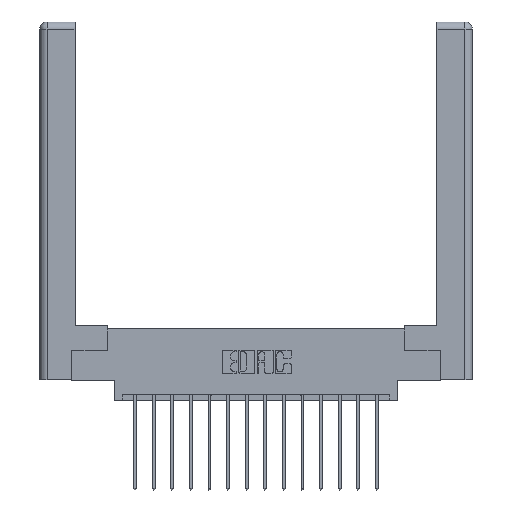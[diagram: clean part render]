
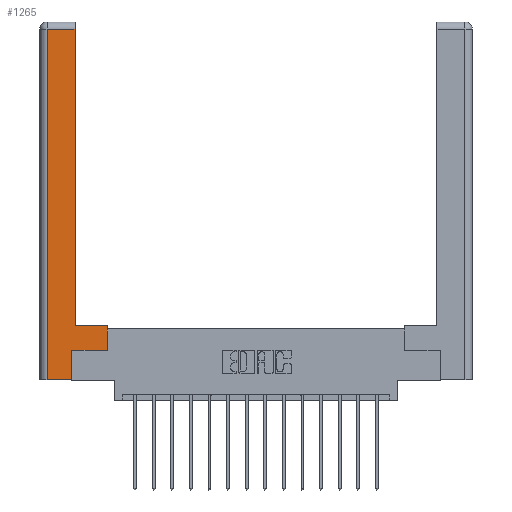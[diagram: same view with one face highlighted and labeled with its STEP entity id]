
A CAD part, top view. The second image highlights one B-rep face of the part: STEP entity #1265.
In plain terms, the highlighted planar face has unit normal (0, 0, 1).
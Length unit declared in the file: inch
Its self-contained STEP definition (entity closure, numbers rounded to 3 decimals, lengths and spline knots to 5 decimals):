
#77 = CARTESIAN_POINT ( 'NONE',  ( 0.0615, 0., 0. ) ) ;
#133 = FACE_OUTER_BOUND ( 'NONE', #11661, .T. ) ;
#338 = VECTOR ( 'NONE', #8718, 39.37008 ) ;
#822 = EDGE_CURVE ( 'NONE', #15724, #2170, #10951, .T. ) ;
#1139 = EDGE_CURVE ( 'NONE', #3528, #12792, #16197, .T. ) ;
#1265 = ADVANCED_FACE ( 'NONE', ( #133 ), #13441, .F. ) ;
#1387 = AXIS2_PLACEMENT_3D ( 'NONE', #4194, #10757, #2815 ) ;
#1439 = ORIENTED_EDGE ( 'NONE', *, *, #4792, .T. ) ;
#1557 = DIRECTION ( 'NONE',  ( 0., 1., 0. ) ) ;
#1636 = CARTESIAN_POINT ( 'NONE',  ( 0.565, 0.245, 0. ) ) ;
#1803 = VECTOR ( 'NONE', #3626, 39.37008 ) ;
#1825 = CARTESIAN_POINT ( 'NONE',  ( 0.265, 0.245, 0. ) ) ;
#2148 = VERTEX_POINT ( 'NONE', #11118 ) ;
#2170 = VERTEX_POINT ( 'NONE', #11792 ) ;
#2693 = CARTESIAN_POINT ( 'NONE',  ( 0.0615, 2.94, 0. ) ) ;
#2815 = DIRECTION ( 'NONE',  ( -1., 0., 0. ) ) ;
#2923 = DIRECTION ( 'NONE',  ( 1., 0., 0. ) ) ;
#3528 = VERTEX_POINT ( 'NONE', #2693 ) ;
#3626 = DIRECTION ( 'NONE',  ( 1., 0., 0. ) ) ;
#3769 = DIRECTION ( 'NONE',  ( 0., -1., 0. ) ) ;
#4194 = CARTESIAN_POINT ( 'NONE',  ( 0., 0., 0. ) ) ;
#4705 = ORIENTED_EDGE ( 'NONE', *, *, #16252, .T. ) ;
#4792 = EDGE_CURVE ( 'NONE', #7617, #15724, #8125, .T. ) ;
#5646 = DIRECTION ( 'NONE',  ( 0., 1., 0. ) ) ;
#6148 = LINE ( 'NONE', #6435, #1803 ) ;
#6435 = CARTESIAN_POINT ( 'NONE',  ( 0.265, 0., 0. ) ) ;
#6750 = VECTOR ( 'NONE', #3769, 39.37008 ) ;
#6788 = ORIENTED_EDGE ( 'NONE', *, *, #10988, .T. ) ;
#7175 = VECTOR ( 'NONE', #16006, 39.37008 ) ;
#7399 = DIRECTION ( 'NONE',  ( 0., 1., 0. ) ) ;
#7617 = VERTEX_POINT ( 'NONE', #1825 ) ;
#8019 = EDGE_CURVE ( 'NONE', #2170, #9097, #10737, .T. ) ;
#8125 = LINE ( 'NONE', #10688, #9578 ) ;
#8718 = DIRECTION ( 'NONE',  ( -1., 0., 0. ) ) ;
#8876 = EDGE_CURVE ( 'NONE', #12792, #12519, #6148, .T. ) ;
#8893 = CARTESIAN_POINT ( 'NONE',  ( 0.0615, 2.94, 0. ) ) ;
#9071 = LINE ( 'NONE', #8893, #338 ) ;
#9097 = VERTEX_POINT ( 'NONE', #9476 ) ;
#9248 = CARTESIAN_POINT ( 'NONE',  ( 0.295, 0.45, 0. ) ) ;
#9427 = EDGE_CURVE ( 'NONE', #2148, #3528, #9071, .T. ) ;
#9476 = CARTESIAN_POINT ( 'NONE',  ( 0.295, 0.45, 0. ) ) ;
#9578 = VECTOR ( 'NONE', #2923, 39.37008 ) ;
#10688 = CARTESIAN_POINT ( 'NONE',  ( 0.565, 0.245, 0. ) ) ;
#10737 = LINE ( 'NONE', #9248, #7175 ) ;
#10757 = DIRECTION ( 'NONE',  ( 0., 0., -1. ) ) ;
#10951 = LINE ( 'NONE', #12166, #11805 ) ;
#10988 = EDGE_CURVE ( 'NONE', #12519, #7617, #15285, .T. ) ;
#11025 = LINE ( 'NONE', #13678, #17116 ) ;
#11093 = VECTOR ( 'NONE', #7399, 39.37008 ) ;
#11118 = CARTESIAN_POINT ( 'NONE',  ( 0.295, 2.94, 0. ) ) ;
#11661 = EDGE_LOOP ( 'NONE', ( #4705, #16142, #13622, #16574, #6788, #1439, #11720, #15894 ) ) ;
#11713 = CARTESIAN_POINT ( 'NONE',  ( 0.265, 0., 0. ) ) ;
#11720 = ORIENTED_EDGE ( 'NONE', *, *, #822, .T. ) ;
#11792 = CARTESIAN_POINT ( 'NONE',  ( 0.565, 0.45, 0. ) ) ;
#11805 = VECTOR ( 'NONE', #1557, 39.37008 ) ;
#12166 = CARTESIAN_POINT ( 'NONE',  ( 0.565, 0.45, 0. ) ) ;
#12519 = VERTEX_POINT ( 'NONE', #11713 ) ;
#12792 = VERTEX_POINT ( 'NONE', #77 ) ;
#12880 = CARTESIAN_POINT ( 'NONE',  ( 0.265, 0.245, 0. ) ) ;
#13249 = CARTESIAN_POINT ( 'NONE',  ( 0.0615, 0., 0. ) ) ;
#13441 = PLANE ( 'NONE',  #1387 ) ;
#13622 = ORIENTED_EDGE ( 'NONE', *, *, #1139, .T. ) ;
#13678 = CARTESIAN_POINT ( 'NONE',  ( 0.295, 3., 0. ) ) ;
#15285 = LINE ( 'NONE', #12880, #11093 ) ;
#15724 = VERTEX_POINT ( 'NONE', #1636 ) ;
#15894 = ORIENTED_EDGE ( 'NONE', *, *, #8019, .T. ) ;
#16006 = DIRECTION ( 'NONE',  ( -1., 0., 0. ) ) ;
#16142 = ORIENTED_EDGE ( 'NONE', *, *, #9427, .T. ) ;
#16197 = LINE ( 'NONE', #13249, #6750 ) ;
#16252 = EDGE_CURVE ( 'NONE', #9097, #2148, #11025, .T. ) ;
#16574 = ORIENTED_EDGE ( 'NONE', *, *, #8876, .T. ) ;
#17116 = VECTOR ( 'NONE', #5646, 39.37008 ) ;
